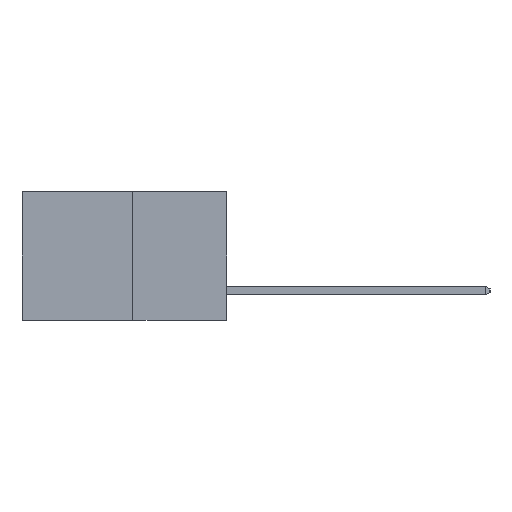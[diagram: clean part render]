
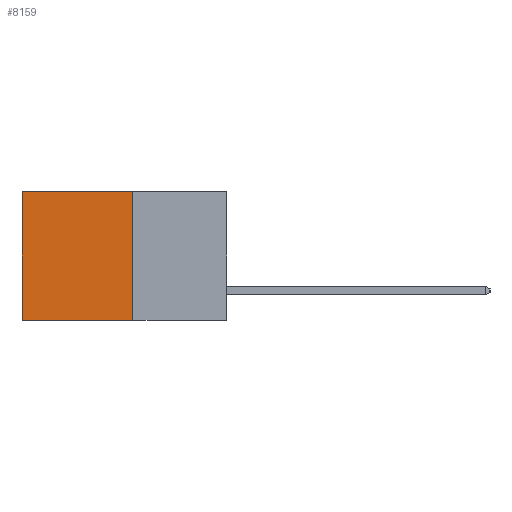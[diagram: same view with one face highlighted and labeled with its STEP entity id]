
A CAD part, left-side view. The second image highlights one B-rep face of the part: STEP entity #8159.
In plain terms, the highlighted planar face has unit normal (-1, 0, 0).
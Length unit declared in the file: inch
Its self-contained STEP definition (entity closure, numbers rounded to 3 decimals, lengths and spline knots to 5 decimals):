
#739 = VERTEX_POINT ( 'NONE', #5386 ) ;
#1013 = ORIENTED_EDGE ( 'NONE', *, *, #8174, .F. ) ;
#1328 = VECTOR ( 'NONE', #7583, 39.37008 ) ;
#1519 = EDGE_CURVE ( 'NONE', #2373, #1763, #2356, .T. ) ;
#1547 = LINE ( 'NONE', #7605, #1328 ) ;
#1593 = CARTESIAN_POINT ( 'NONE',  ( 0.277, 0.27, 0. ) ) ;
#1649 = CARTESIAN_POINT ( 'NONE',  ( 0.277, 0.59, -0.37 ) ) ;
#1712 = DIRECTION ( 'NONE',  ( 0., 1., 0. ) ) ;
#1763 = VERTEX_POINT ( 'NONE', #5307 ) ;
#2072 = AXIS2_PLACEMENT_3D ( 'NONE', #6000, #5992, #5983 ) ;
#2356 = LINE ( 'NONE', #1593, #3411 ) ;
#2373 = VERTEX_POINT ( 'NONE', #7969 ) ;
#2530 = LINE ( 'NONE', #1649, #7496 ) ;
#2621 = VECTOR ( 'NONE', #5864, 39.37008 ) ;
#2662 = EDGE_LOOP ( 'NONE', ( #6348, #7524, #1013, #6826 ) ) ;
#2962 = EDGE_CURVE ( 'NONE', #1763, #3937, #2530, .T. ) ;
#3411 = VECTOR ( 'NONE', #1712, 39.37008 ) ;
#3435 = DIRECTION ( 'NONE',  ( 0., 0., -1. ) ) ;
#3937 = VERTEX_POINT ( 'NONE', #4577 ) ;
#4209 = LINE ( 'NONE', #5958, #2621 ) ;
#4577 = CARTESIAN_POINT ( 'NONE',  ( 0.277, 0.59, -0.37 ) ) ;
#5307 = CARTESIAN_POINT ( 'NONE',  ( 0.277, 0.59, 0. ) ) ;
#5386 = CARTESIAN_POINT ( 'NONE',  ( 0.277, 0.27, -0.37 ) ) ;
#5864 = DIRECTION ( 'NONE',  ( 0., 0., -1. ) ) ;
#5958 = CARTESIAN_POINT ( 'NONE',  ( 0.277, 0.27, -0.37 ) ) ;
#5983 = DIRECTION ( 'NONE',  ( 0., 0., -1. ) ) ;
#5992 = DIRECTION ( 'NONE',  ( 1., 0., 0. ) ) ;
#6000 = CARTESIAN_POINT ( 'NONE',  ( 0.277, 0.27, -0.37 ) ) ;
#6004 = PLANE ( 'NONE',  #2072 ) ;
#6348 = ORIENTED_EDGE ( 'NONE', *, *, #2962, .T. ) ;
#6826 = ORIENTED_EDGE ( 'NONE', *, *, #1519, .T. ) ;
#7496 = VECTOR ( 'NONE', #3435, 39.37008 ) ;
#7524 = ORIENTED_EDGE ( 'NONE', *, *, #7737, .F. ) ;
#7583 = DIRECTION ( 'NONE',  ( 0., 1., 0. ) ) ;
#7605 = CARTESIAN_POINT ( 'NONE',  ( 0.277, 0.27, -0.37 ) ) ;
#7737 = EDGE_CURVE ( 'NONE', #739, #3937, #1547, .T. ) ;
#7781 = FACE_OUTER_BOUND ( 'NONE', #2662, .T. ) ;
#7969 = CARTESIAN_POINT ( 'NONE',  ( 0.277, 0.27, 0. ) ) ;
#8159 = ADVANCED_FACE ( 'NONE', ( #7781 ), #6004, .F. ) ;
#8174 = EDGE_CURVE ( 'NONE', #2373, #739, #4209, .T. ) ;
